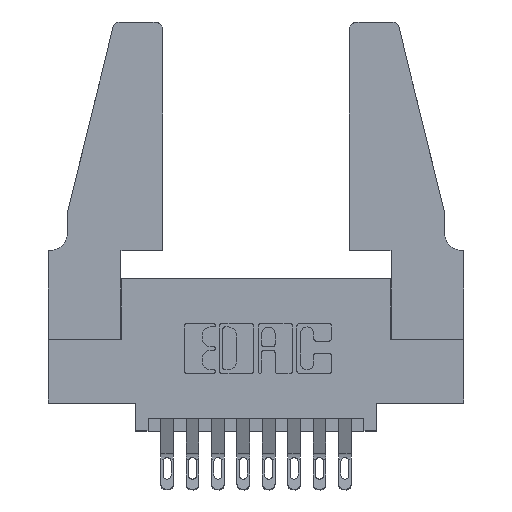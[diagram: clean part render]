
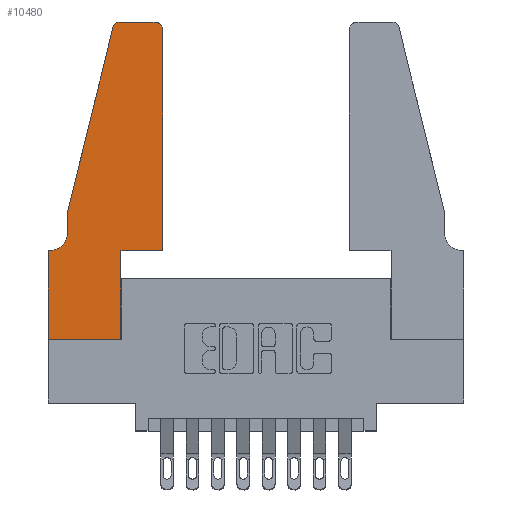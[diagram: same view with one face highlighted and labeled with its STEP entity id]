
A CAD part, top view. The second image highlights one B-rep face of the part: STEP entity #10480.
In plain terms, the highlighted planar face has unit normal (0, 0, 1).
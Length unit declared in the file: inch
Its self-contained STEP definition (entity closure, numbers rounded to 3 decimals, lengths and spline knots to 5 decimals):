
#12 = ORIENTED_EDGE ( 'NONE', *, *, #6090, .T. ) ;
#273 = ORIENTED_EDGE ( 'NONE', *, *, #1597, .T. ) ;
#291 = CARTESIAN_POINT ( 'NONE',  ( 0.25487, 1.22718, 0.37 ) ) ;
#570 = CARTESIAN_POINT ( 'NONE',  ( 0.0755, 0.42, 0.37 ) ) ;
#643 = AXIS2_PLACEMENT_3D ( 'NONE', #12589, #9492, #11625 ) ;
#844 = VERTEX_POINT ( 'NONE', #12974 ) ;
#1062 = LINE ( 'NONE', #1986, #9355 ) ;
#1327 = ORIENTED_EDGE ( 'NONE', *, *, #12010, .T. ) ;
#1418 = VERTEX_POINT ( 'NONE', #291 ) ;
#1597 = EDGE_CURVE ( 'NONE', #5502, #2078, #9078, .T. ) ;
#1669 = VERTEX_POINT ( 'NONE', #11512 ) ;
#1986 = CARTESIAN_POINT ( 'NONE',  ( 0.2605, 1.25, 0.37 ) ) ;
#2078 = VERTEX_POINT ( 'NONE', #7903 ) ;
#2167 = DIRECTION ( 'NONE',  ( 1., 0., 0. ) ) ;
#2229 = EDGE_CURVE ( 'NONE', #9652, #844, #12660, .T. ) ;
#2245 = AXIS2_PLACEMENT_3D ( 'NONE', #3509, #10723, #5471 ) ;
#2304 = AXIS2_PLACEMENT_3D ( 'NONE', #8829, #3556, #3812 ) ;
#2391 = CARTESIAN_POINT ( 'NONE',  ( 0.0055, 0.35, 0.37 ) ) ;
#2488 = CARTESIAN_POINT ( 'NONE',  ( 0.4205, 1.25, 0.37 ) ) ;
#2779 = VERTEX_POINT ( 'NONE', #12610 ) ;
#2868 = DIRECTION ( 'NONE',  ( 0., 1., 0. ) ) ;
#2877 = VECTOR ( 'NONE', #2868, 39.37008 ) ;
#3267 = EDGE_CURVE ( 'NONE', #8907, #7735, #5594, .T. ) ;
#3489 = ORIENTED_EDGE ( 'NONE', *, *, #7908, .T. ) ;
#3509 = CARTESIAN_POINT ( 'NONE',  ( 0., 0.35, 0.37 ) ) ;
#3556 = DIRECTION ( 'NONE',  ( 0., 0., 1. ) ) ;
#3715 = LINE ( 'NONE', #11837, #7459 ) ;
#3812 = DIRECTION ( 'NONE',  ( 1., 0., 0. ) ) ;
#3989 = VERTEX_POINT ( 'NONE', #8763 ) ;
#4397 = ORIENTED_EDGE ( 'NONE', *, *, #3267, .T. ) ;
#4401 = ORIENTED_EDGE ( 'NONE', *, *, #7930, .T. ) ;
#4431 = VECTOR ( 'NONE', #6655, 39.37008 ) ;
#4469 = CARTESIAN_POINT ( 'NONE',  ( 0.0755, 0.5, 0.37 ) ) ;
#4816 = ORIENTED_EDGE ( 'NONE', *, *, #12876, .T. ) ;
#4961 = EDGE_CURVE ( 'NONE', #1418, #9564, #9990, .T. ) ;
#4972 = DIRECTION ( 'NONE',  ( 1., 0., 0. ) ) ;
#5137 = DIRECTION ( 'NONE',  ( 0., 1., 0. ) ) ;
#5189 = VECTOR ( 'NONE', #12817, 39.37008 ) ;
#5456 = CARTESIAN_POINT ( 'NONE',  ( 0.0755, 0.35, 0.37 ) ) ;
#5471 = DIRECTION ( 'NONE',  ( 1., 0., 0. ) ) ;
#5496 = CARTESIAN_POINT ( 'NONE',  ( 0.0755, 0.5, 0.37 ) ) ;
#5502 = VERTEX_POINT ( 'NONE', #8453 ) ;
#5578 = FACE_OUTER_BOUND ( 'NONE', #5945, .T. ) ;
#5594 = CIRCLE ( 'NONE', #7800, 0.07 ) ;
#5822 = EDGE_CURVE ( 'NONE', #9564, #8907, #7986, .T. ) ;
#5889 = DIRECTION ( 'NONE',  ( 0., -1., 0. ) ) ;
#5945 = EDGE_LOOP ( 'NONE', ( #4816, #12, #8188, #9997, #4397, #7217, #3489, #4401, #7690, #10484, #273, #1327 ) ) ;
#6030 = DIRECTION ( 'NONE',  ( -1., 0., 0. ) ) ;
#6090 = EDGE_CURVE ( 'NONE', #3989, #1418, #8812, .T. ) ;
#6290 = VECTOR ( 'NONE', #5137, 39.37008 ) ;
#6573 = EDGE_CURVE ( 'NONE', #844, #5502, #13052, .T. ) ;
#6584 = LINE ( 'NONE', #5456, #7229 ) ;
#6655 = DIRECTION ( 'NONE',  ( -0.239, -0.971, 0. ) ) ;
#7123 = LINE ( 'NONE', #12473, #10740 ) ;
#7217 = ORIENTED_EDGE ( 'NONE', *, *, #10628, .T. ) ;
#7229 = VECTOR ( 'NONE', #12684, 39.37008 ) ;
#7355 = CARTESIAN_POINT ( 'NONE',  ( 0.2865, 0.35, 0.37 ) ) ;
#7459 = VECTOR ( 'NONE', #5889, 39.37008 ) ;
#7522 = CARTESIAN_POINT ( 'NONE',  ( 0.0755, 0.5, 0.37 ) ) ;
#7690 = ORIENTED_EDGE ( 'NONE', *, *, #2229, .T. ) ;
#7735 = VERTEX_POINT ( 'NONE', #2391 ) ;
#7800 = AXIS2_PLACEMENT_3D ( 'NONE', #12455, #10326, #13413 ) ;
#7903 = CARTESIAN_POINT ( 'NONE',  ( 0.4505, 1.22, 0.37 ) ) ;
#7908 = EDGE_CURVE ( 'NONE', #2779, #1669, #3715, .T. ) ;
#7930 = EDGE_CURVE ( 'NONE', #1669, #9652, #7123, .T. ) ;
#7986 = LINE ( 'NONE', #7522, #5189 ) ;
#8188 = ORIENTED_EDGE ( 'NONE', *, *, #4961, .T. ) ;
#8453 = CARTESIAN_POINT ( 'NONE',  ( 0.4505, 0.35, 0.37 ) ) ;
#8604 = PLANE ( 'NONE',  #2245 ) ;
#8763 = CARTESIAN_POINT ( 'NONE',  ( 0.284, 1.25, 0.37 ) ) ;
#8812 = CIRCLE ( 'NONE', #2304, 0.03 ) ;
#8829 = CARTESIAN_POINT ( 'NONE',  ( 0.284, 1.22, 0.37 ) ) ;
#8907 = VERTEX_POINT ( 'NONE', #570 ) ;
#9078 = LINE ( 'NONE', #10137, #6290 ) ;
#9182 = VERTEX_POINT ( 'NONE', #2488 ) ;
#9355 = VECTOR ( 'NONE', #6030, 39.37008 ) ;
#9492 = DIRECTION ( 'NONE',  ( 0., 0., 1. ) ) ;
#9564 = VERTEX_POINT ( 'NONE', #5496 ) ;
#9652 = VERTEX_POINT ( 'NONE', #10177 ) ;
#9815 = CIRCLE ( 'NONE', #643, 0.03 ) ;
#9883 = CARTESIAN_POINT ( 'NONE',  ( 0.4505, 0.35, 0.37 ) ) ;
#9990 = LINE ( 'NONE', #4469, #4431 ) ;
#9997 = ORIENTED_EDGE ( 'NONE', *, *, #5822, .T. ) ;
#10137 = CARTESIAN_POINT ( 'NONE',  ( 0.4505, 0.35, 0.37 ) ) ;
#10177 = CARTESIAN_POINT ( 'NONE',  ( 0.2865, 0., 0.37 ) ) ;
#10326 = DIRECTION ( 'NONE',  ( 0., 0., -1. ) ) ;
#10480 = ADVANCED_FACE ( 'NONE', ( #5578 ), #8604, .T. ) ;
#10484 = ORIENTED_EDGE ( 'NONE', *, *, #6573, .T. ) ;
#10628 = EDGE_CURVE ( 'NONE', #7735, #2779, #6584, .T. ) ;
#10723 = DIRECTION ( 'NONE',  ( 0., 0., 1. ) ) ;
#10740 = VECTOR ( 'NONE', #2167, 39.37008 ) ;
#11512 = CARTESIAN_POINT ( 'NONE',  ( 0., 0., 0.37 ) ) ;
#11625 = DIRECTION ( 'NONE',  ( 1., 0., 0. ) ) ;
#11837 = CARTESIAN_POINT ( 'NONE',  ( 0., 0., 0.37 ) ) ;
#12010 = EDGE_CURVE ( 'NONE', #2078, #9182, #9815, .T. ) ;
#12455 = CARTESIAN_POINT ( 'NONE',  ( 0.0055, 0.42, 0.37 ) ) ;
#12473 = CARTESIAN_POINT ( 'NONE',  ( 0., 0., 0.37 ) ) ;
#12589 = CARTESIAN_POINT ( 'NONE',  ( 0.4205, 1.22, 0.37 ) ) ;
#12610 = CARTESIAN_POINT ( 'NONE',  ( 0., 0.35, 0.37 ) ) ;
#12660 = LINE ( 'NONE', #7355, #2877 ) ;
#12684 = DIRECTION ( 'NONE',  ( -1., 0., 0. ) ) ;
#12817 = DIRECTION ( 'NONE',  ( 0., -1., 0. ) ) ;
#12876 = EDGE_CURVE ( 'NONE', #9182, #3989, #1062, .T. ) ;
#12888 = VECTOR ( 'NONE', #4972, 39.37008 ) ;
#12974 = CARTESIAN_POINT ( 'NONE',  ( 0.2865, 0.35, 0.37 ) ) ;
#13052 = LINE ( 'NONE', #9883, #12888 ) ;
#13413 = DIRECTION ( 'NONE',  ( -1., 0., 0. ) ) ;
